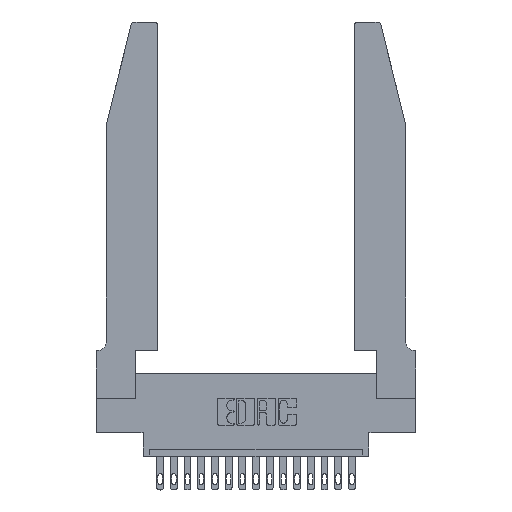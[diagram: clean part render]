
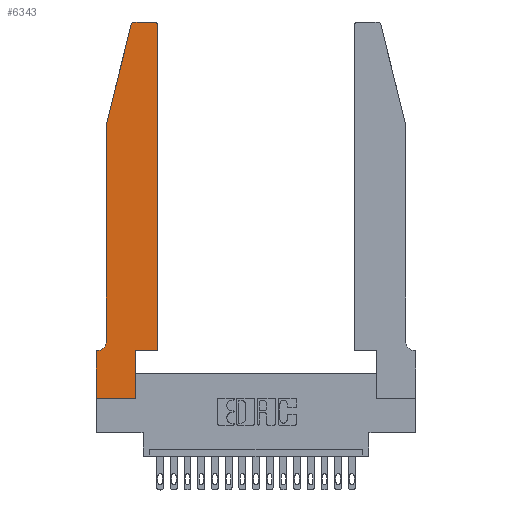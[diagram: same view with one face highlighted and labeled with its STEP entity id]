
A CAD part, top view. The second image highlights one B-rep face of the part: STEP entity #6343.
In plain terms, the highlighted planar face has unit normal (0, 0, 1).
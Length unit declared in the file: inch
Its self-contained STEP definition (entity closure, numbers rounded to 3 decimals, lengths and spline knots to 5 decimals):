
#73 = EDGE_CURVE ( 'NONE', #11892, #5909, #3365, .T. ) ;
#81 = CARTESIAN_POINT ( 'NONE',  ( 0.4505, 0.35, 0.37 ) ) ;
#121 = CARTESIAN_POINT ( 'NONE',  ( 0.4205, 2.75, 0.37 ) ) ;
#888 = ORIENTED_EDGE ( 'NONE', *, *, #8845, .T. ) ;
#995 = DIRECTION ( 'NONE',  ( 0., 0., 1. ) ) ;
#1103 = CARTESIAN_POINT ( 'NONE',  ( 0.284, 2.72, 0.37 ) ) ;
#1292 = DIRECTION ( 'NONE',  ( 1., 0., 0. ) ) ;
#1640 = ORIENTED_EDGE ( 'NONE', *, *, #2047, .T. ) ;
#1809 = VERTEX_POINT ( 'NONE', #18834 ) ;
#2047 = EDGE_CURVE ( 'NONE', #12341, #1809, #13288, .T. ) ;
#2342 = CARTESIAN_POINT ( 'NONE',  ( 0.4205, 2.72, 0.37 ) ) ;
#2396 = DIRECTION ( 'NONE',  ( -1., 0., 0. ) ) ;
#2526 = DIRECTION ( 'NONE',  ( -1., 0., 0. ) ) ;
#2613 = ORIENTED_EDGE ( 'NONE', *, *, #7902, .T. ) ;
#2616 = CARTESIAN_POINT ( 'NONE',  ( 0.4505, 2.72, 0.37 ) ) ;
#2823 = LINE ( 'NONE', #81, #4267 ) ;
#2834 = PLANE ( 'NONE',  #11947 ) ;
#3135 = DIRECTION ( 'NONE',  ( 1., 0., 0. ) ) ;
#3302 = ORIENTED_EDGE ( 'NONE', *, *, #10143, .T. ) ;
#3365 = LINE ( 'NONE', #6899, #5477 ) ;
#3399 = EDGE_CURVE ( 'NONE', #1809, #9517, #17538, .T. ) ;
#3557 = VECTOR ( 'NONE', #13348, 39.37008 ) ;
#3937 = LINE ( 'NONE', #9904, #8481 ) ;
#3971 = DIRECTION ( 'NONE',  ( 1., 0., 0. ) ) ;
#4010 = LINE ( 'NONE', #15635, #8550 ) ;
#4187 = LINE ( 'NONE', #14491, #8035 ) ;
#4267 = VECTOR ( 'NONE', #18492, 39.37008 ) ;
#4274 = DIRECTION ( 'NONE',  ( 0., -1., 0. ) ) ;
#4689 = CARTESIAN_POINT ( 'NONE',  ( 0., 0., 0.37 ) ) ;
#4921 = CIRCLE ( 'NONE', #13845, 0.07 ) ;
#5038 = DIRECTION ( 'NONE',  ( 0., 1., 0. ) ) ;
#5181 = ORIENTED_EDGE ( 'NONE', *, *, #3399, .T. ) ;
#5347 = DIRECTION ( 'NONE',  ( 1., 0., 0. ) ) ;
#5477 = VECTOR ( 'NONE', #17384, 39.37008 ) ;
#5738 = CARTESIAN_POINT ( 'NONE',  ( 0.0755, 0.35, 0.37 ) ) ;
#5909 = VERTEX_POINT ( 'NONE', #4689 ) ;
#6343 = ADVANCED_FACE ( 'NONE', ( #10066 ), #2834, .T. ) ;
#6527 = AXIS2_PLACEMENT_3D ( 'NONE', #1103, #8945, #1292 ) ;
#6899 = CARTESIAN_POINT ( 'NONE',  ( 0., 0., 0.37 ) ) ;
#7197 = EDGE_CURVE ( 'NONE', #19273, #16414, #2823, .T. ) ;
#7212 = CARTESIAN_POINT ( 'NONE',  ( 0.0755, 0.42, 0.37 ) ) ;
#7345 = LINE ( 'NONE', #16360, #3557 ) ;
#7499 = CARTESIAN_POINT ( 'NONE',  ( 0.25487, 2.72718, 0.37 ) ) ;
#7500 = EDGE_CURVE ( 'NONE', #16414, #12753, #7345, .T. ) ;
#7516 = ORIENTED_EDGE ( 'NONE', *, *, #7197, .T. ) ;
#7534 = VERTEX_POINT ( 'NONE', #7212 ) ;
#7902 = EDGE_CURVE ( 'NONE', #18689, #19273, #4010, .T. ) ;
#8035 = VECTOR ( 'NONE', #5347, 39.37008 ) ;
#8149 = CIRCLE ( 'NONE', #13474, 0.03 ) ;
#8481 = VECTOR ( 'NONE', #17535, 39.37008 ) ;
#8550 = VECTOR ( 'NONE', #5038, 39.37008 ) ;
#8845 = EDGE_CURVE ( 'NONE', #9839, #11892, #12592, .T. ) ;
#8945 = DIRECTION ( 'NONE',  ( 0., 0., 1. ) ) ;
#9277 = VECTOR ( 'NONE', #12248, 39.37008 ) ;
#9517 = VERTEX_POINT ( 'NONE', #7499 ) ;
#9839 = VERTEX_POINT ( 'NONE', #10333 ) ;
#9904 = CARTESIAN_POINT ( 'NONE',  ( 0.0755, 2., 0.37 ) ) ;
#9926 = CARTESIAN_POINT ( 'NONE',  ( 0.2865, 0., 0.37 ) ) ;
#10066 = FACE_OUTER_BOUND ( 'NONE', #13425, .T. ) ;
#10107 = EDGE_CURVE ( 'NONE', #7534, #9839, #4921, .T. ) ;
#10143 = EDGE_CURVE ( 'NONE', #5909, #18689, #4187, .T. ) ;
#10333 = CARTESIAN_POINT ( 'NONE',  ( 0.0055, 0.35, 0.37 ) ) ;
#10494 = CARTESIAN_POINT ( 'NONE',  ( 0., 0.35, 0.37 ) ) ;
#10754 = CARTESIAN_POINT ( 'NONE',  ( 0.2605, 2.75, 0.37 ) ) ;
#11377 = CARTESIAN_POINT ( 'NONE',  ( 0., 0.35, 0.37 ) ) ;
#11411 = DIRECTION ( 'NONE',  ( 0., 0., 1. ) ) ;
#11892 = VERTEX_POINT ( 'NONE', #11377 ) ;
#11947 = AXIS2_PLACEMENT_3D ( 'NONE', #10494, #11411, #3135 ) ;
#12228 = ORIENTED_EDGE ( 'NONE', *, *, #10107, .T. ) ;
#12248 = DIRECTION ( 'NONE',  ( -1., 0., 0. ) ) ;
#12341 = VERTEX_POINT ( 'NONE', #121 ) ;
#12353 = LINE ( 'NONE', #17930, #16161 ) ;
#12570 = ORIENTED_EDGE ( 'NONE', *, *, #13047, .T. ) ;
#12592 = LINE ( 'NONE', #5738, #14714 ) ;
#12617 = VERTEX_POINT ( 'NONE', #19245 ) ;
#12753 = VERTEX_POINT ( 'NONE', #2616 ) ;
#12963 = DIRECTION ( 'NONE',  ( 0., 0., -1. ) ) ;
#13047 = EDGE_CURVE ( 'NONE', #12753, #12341, #8149, .T. ) ;
#13288 = LINE ( 'NONE', #10754, #9277 ) ;
#13348 = DIRECTION ( 'NONE',  ( 0., 1., 0. ) ) ;
#13425 = EDGE_LOOP ( 'NONE', ( #1640, #5181, #14278, #17392, #12228, #888, #15863, #3302, #2613, #7516, #14005, #12570 ) ) ;
#13474 = AXIS2_PLACEMENT_3D ( 'NONE', #2342, #995, #3971 ) ;
#13845 = AXIS2_PLACEMENT_3D ( 'NONE', #14684, #12963, #2396 ) ;
#14005 = ORIENTED_EDGE ( 'NONE', *, *, #7500, .T. ) ;
#14278 = ORIENTED_EDGE ( 'NONE', *, *, #17039, .T. ) ;
#14491 = CARTESIAN_POINT ( 'NONE',  ( 0., 0., 0.37 ) ) ;
#14684 = CARTESIAN_POINT ( 'NONE',  ( 0.0055, 0.42, 0.37 ) ) ;
#14714 = VECTOR ( 'NONE', #2526, 39.37008 ) ;
#14725 = CARTESIAN_POINT ( 'NONE',  ( 0.2865, 0.35, 0.37 ) ) ;
#14788 = EDGE_CURVE ( 'NONE', #12617, #7534, #12353, .T. ) ;
#15618 = CARTESIAN_POINT ( 'NONE',  ( 0.4505, 0.35, 0.37 ) ) ;
#15635 = CARTESIAN_POINT ( 'NONE',  ( 0.2865, 0.35, 0.37 ) ) ;
#15863 = ORIENTED_EDGE ( 'NONE', *, *, #73, .T. ) ;
#16161 = VECTOR ( 'NONE', #4274, 39.37008 ) ;
#16360 = CARTESIAN_POINT ( 'NONE',  ( 0.4505, 0.35, 0.37 ) ) ;
#16414 = VERTEX_POINT ( 'NONE', #15618 ) ;
#17039 = EDGE_CURVE ( 'NONE', #9517, #12617, #3937, .T. ) ;
#17384 = DIRECTION ( 'NONE',  ( 0., -1., 0. ) ) ;
#17392 = ORIENTED_EDGE ( 'NONE', *, *, #14788, .T. ) ;
#17535 = DIRECTION ( 'NONE',  ( -0.239, -0.971, 0. ) ) ;
#17538 = CIRCLE ( 'NONE', #6527, 0.03 ) ;
#17930 = CARTESIAN_POINT ( 'NONE',  ( 0.0755, 2., 0.37 ) ) ;
#18492 = DIRECTION ( 'NONE',  ( 1., 0., 0. ) ) ;
#18689 = VERTEX_POINT ( 'NONE', #9926 ) ;
#18834 = CARTESIAN_POINT ( 'NONE',  ( 0.284, 2.75, 0.37 ) ) ;
#19245 = CARTESIAN_POINT ( 'NONE',  ( 0.0755, 2., 0.37 ) ) ;
#19273 = VERTEX_POINT ( 'NONE', #14725 ) ;
